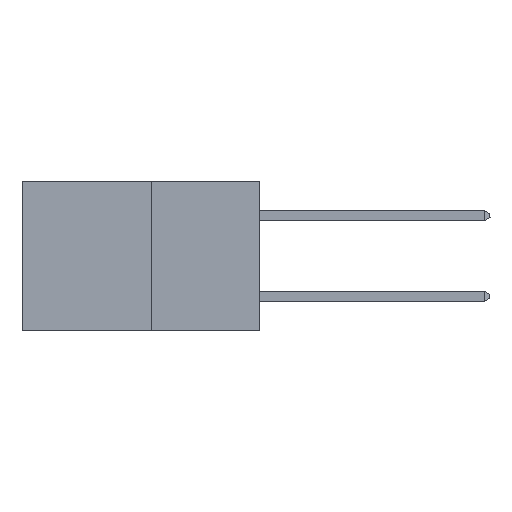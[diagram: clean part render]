
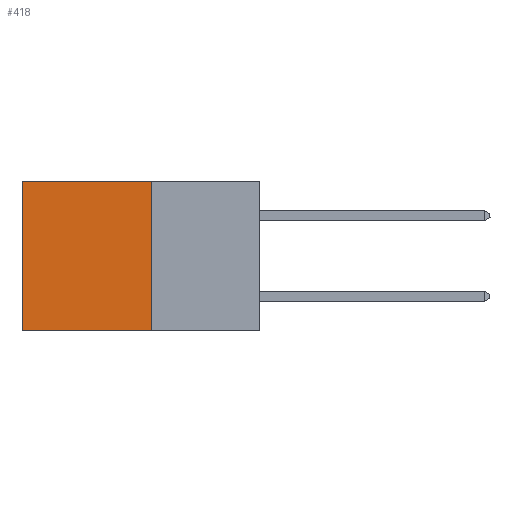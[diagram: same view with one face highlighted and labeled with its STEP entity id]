
A CAD part, left-side view. The second image highlights one B-rep face of the part: STEP entity #418.
In plain terms, the highlighted planar face has unit normal (-1, 0, 0).
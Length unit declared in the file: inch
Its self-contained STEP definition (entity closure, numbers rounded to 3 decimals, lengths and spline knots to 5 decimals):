
#52 = DIRECTION ( 'NONE',  ( 0., 0., -1. ) ) ;
#418 = ADVANCED_FACE ( 'NONE', ( #22676 ), #20649, .F. ) ;
#968 = VECTOR ( 'NONE', #27819, 39.37008 ) ;
#2258 = LINE ( 'NONE', #17934, #14115 ) ;
#2853 = ORIENTED_EDGE ( 'NONE', *, *, #3439, .T. ) ;
#3200 = ORIENTED_EDGE ( 'NONE', *, *, #16388, .F. ) ;
#3439 = EDGE_CURVE ( 'NONE', #17497, #3847, #2258, .T. ) ;
#3847 = VERTEX_POINT ( 'NONE', #7477 ) ;
#5986 = CARTESIAN_POINT ( 'NONE',  ( 0.277, 0.27, -0.37 ) ) ;
#6871 = VERTEX_POINT ( 'NONE', #5986 ) ;
#6905 = CARTESIAN_POINT ( 'NONE',  ( 0.277, 0.27, 0. ) ) ;
#7313 = CARTESIAN_POINT ( 'NONE',  ( 0.277, 0.27, -0.37 ) ) ;
#7477 = CARTESIAN_POINT ( 'NONE',  ( 0.277, 0.59, -0.37 ) ) ;
#8305 = LINE ( 'NONE', #24566, #26859 ) ;
#9661 = DIRECTION ( 'NONE',  ( 0., 1., 0. ) ) ;
#10578 = DIRECTION ( 'NONE',  ( 0., 0., -1. ) ) ;
#10607 = VECTOR ( 'NONE', #9661, 39.37008 ) ;
#12267 = EDGE_LOOP ( 'NONE', ( #2853, #3200, #13764, #29941 ) ) ;
#13764 = ORIENTED_EDGE ( 'NONE', *, *, #23883, .F. ) ;
#14115 = VECTOR ( 'NONE', #16765, 39.37008 ) ;
#15030 = LINE ( 'NONE', #6905, #968 ) ;
#16298 = EDGE_CURVE ( 'NONE', #26624, #17497, #15030, .T. ) ;
#16388 = EDGE_CURVE ( 'NONE', #6871, #3847, #23083, .T. ) ;
#16765 = DIRECTION ( 'NONE',  ( 0., 0., -1. ) ) ;
#17497 = VERTEX_POINT ( 'NONE', #20467 ) ;
#17934 = CARTESIAN_POINT ( 'NONE',  ( 0.277, 0.59, -0.37 ) ) ;
#19343 = AXIS2_PLACEMENT_3D ( 'NONE', #30105, #21134, #52 ) ;
#20467 = CARTESIAN_POINT ( 'NONE',  ( 0.277, 0.59, 0. ) ) ;
#20649 = PLANE ( 'NONE',  #19343 ) ;
#21134 = DIRECTION ( 'NONE',  ( 1., 0., 0. ) ) ;
#22676 = FACE_OUTER_BOUND ( 'NONE', #12267, .T. ) ;
#23083 = LINE ( 'NONE', #7313, #10607 ) ;
#23883 = EDGE_CURVE ( 'NONE', #26624, #6871, #8305, .T. ) ;
#24566 = CARTESIAN_POINT ( 'NONE',  ( 0.277, 0.27, -0.37 ) ) ;
#26624 = VERTEX_POINT ( 'NONE', #29909 ) ;
#26859 = VECTOR ( 'NONE', #10578, 39.37008 ) ;
#27819 = DIRECTION ( 'NONE',  ( 0., 1., 0. ) ) ;
#29909 = CARTESIAN_POINT ( 'NONE',  ( 0.277, 0.27, 0. ) ) ;
#29941 = ORIENTED_EDGE ( 'NONE', *, *, #16298, .T. ) ;
#30105 = CARTESIAN_POINT ( 'NONE',  ( 0.277, 0.27, -0.37 ) ) ;
